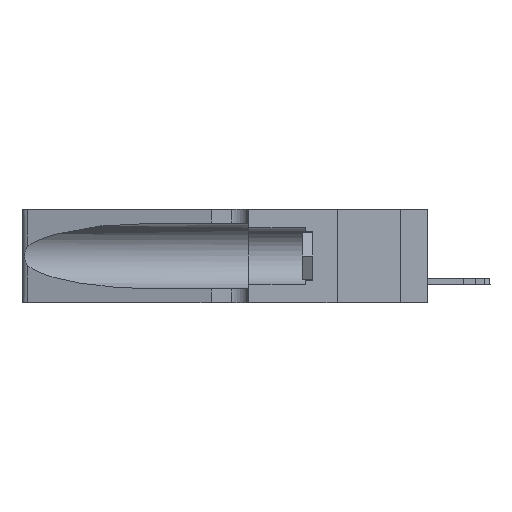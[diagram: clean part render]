
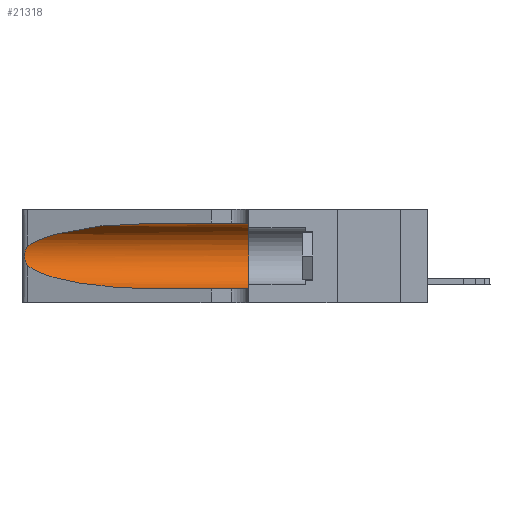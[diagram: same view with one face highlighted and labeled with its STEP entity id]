
A CAD part, left-side view. The second image highlights one B-rep face of the part: STEP entity #21318.
In plain terms, the highlighted cylindrical face has radius 3.308 mm (diameter 6.617 mm), a partial arc.
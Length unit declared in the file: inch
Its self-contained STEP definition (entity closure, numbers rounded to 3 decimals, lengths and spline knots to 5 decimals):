
#778 = DIRECTION ( 'NONE',  ( 0., 0., -1. ) ) ;
#1461 = ORIENTED_EDGE ( 'NONE', *, *, #19994, .F. ) ;
#2462 = CARTESIAN_POINT ( 'NONE',  ( 0.25555, 1.22994, 0.2215 ) ) ;
#2542 = EDGE_LOOP ( 'NONE', ( #11237, #21439, #19529, #3447, #18227, #1461 ) ) ;
#3447 = ORIENTED_EDGE ( 'NONE', *, *, #7201, .T. ) ;
#3636 =( BOUNDED_CURVE ( )  B_SPLINE_CURVE ( 3, ( #21486, #7838, #14524, #28552 ),
 .UNSPECIFIED., .F., .T. ) 
 B_SPLINE_CURVE_WITH_KNOTS ( ( 4, 4 ),
 ( 3.44316, 4.71239 ),
 .UNSPECIFIED. ) 
 CURVE ( )  GEOMETRIC_REPRESENTATION_ITEM ( )  RATIONAL_B_SPLINE_CURVE ( ( 1., 0.87, 0.87, 1. ) ) 
 REPRESENTATION_ITEM ( '' )  );
#3967 = CARTESIAN_POINT ( 'NONE',  ( 0.1305, 1.61858, 0.05475 ) ) ;
#4089 = VECTOR ( 'NONE', #28942, 39.37008 ) ;
#4454 = CARTESIAN_POINT ( 'NONE',  ( 0.26075, 1.23896, 0.19203 ) ) ;
#4654 = CARTESIAN_POINT ( 'NONE',  ( 0.25856, 1.23593, 0.16098 ) ) ;
#5069 = CARTESIAN_POINT ( 'NONE',  ( 0.1305, 1.61858, 0.185 ) ) ;
#5855 = EDGE_CURVE ( 'NONE', #16248, #21308, #26075, .T. ) ;
#6386 = DIRECTION ( 'NONE',  ( 0., 0., 1. ) ) ;
#6632 = CARTESIAN_POINT ( 'NONE',  ( 0.25555, 1.22993, 0.14849 ) ) ;
#6723 = CARTESIAN_POINT ( 'NONE',  ( 0.25487, 1.22718, 0.14631 ) ) ;
#6805 = CARTESIAN_POINT ( 'NONE',  ( 0.25639, 1.23184, 0.21858 ) ) ;
#7201 = EDGE_CURVE ( 'NONE', #9425, #27850, #24384, .T. ) ;
#7838 = CARTESIAN_POINT ( 'NONE',  ( 0.2373, 1.15595, 0.08982 ) ) ;
#8885 = DIRECTION ( 'NONE',  ( 0., -1., 0. ) ) ;
#9065 = CARTESIAN_POINT ( 'NONE',  ( 0.26075, 1.23896, 0.178 ) ) ;
#9425 = VERTEX_POINT ( 'NONE', #17817 ) ;
#10234 = CARTESIAN_POINT ( 'NONE',  ( 0.1305, 0.72297, 0.31525 ) ) ;
#10511 = FACE_OUTER_BOUND ( 'NONE', #2542, .T. ) ;
#11189 = CARTESIAN_POINT ( 'NONE',  ( 0.26017, 1.23833, 0.17102 ) ) ;
#11237 = ORIENTED_EDGE ( 'NONE', *, *, #5855, .T. ) ;
#11334 = LINE ( 'NONE', #22161, #24162 ) ;
#11467 = CARTESIAN_POINT ( 'NONE',  ( 0.25487, 1.22718, 0.22369 ) ) ;
#12929 = B_SPLINE_CURVE_WITH_KNOTS ( 'NONE', 3,
 ( #11467, #2462, #6805, #24854, #22745, #22837, #4454, #9065, #11189, #4654, #27420, #28531, #6632, #6723 ),
 .UNSPECIFIED., .F., .F.,
 ( 4, 2, 2, 2, 2, 2, 4 ),
 ( 0., 0.00027, 0.00053, 0.00107, 0.0016, 0.00187, 0.00214 ),
 .UNSPECIFIED. ) ;
#13054 = DIRECTION ( 'NONE',  ( 0., 1., 0. ) ) ;
#13396 = VERTEX_POINT ( 'NONE', #27294 ) ;
#14204 = CARTESIAN_POINT ( 'NONE',  ( 0.25487, 1.22718, 0.22369 ) ) ;
#14524 = CARTESIAN_POINT ( 'NONE',  ( 0.18966, 0.96281, 0.05475 ) ) ;
#15119 = CARTESIAN_POINT ( 'NONE',  ( 0.25487, 1.22718, 0.22369 ) ) ;
#15885 = CARTESIAN_POINT ( 'NONE',  ( 0.1305, 0.72297, 0.31525 ) ) ;
#16248 = VERTEX_POINT ( 'NONE', #15885 ) ;
#16479 = DIRECTION ( 'NONE',  ( 0., -1., 0. ) ) ;
#16661 = EDGE_CURVE ( 'NONE', #17924, #27850, #25349, .T. ) ;
#17817 = CARTESIAN_POINT ( 'NONE',  ( 0.1305, 0.72297, 0.05475 ) ) ;
#17924 = VERTEX_POINT ( 'NONE', #22054 ) ;
#18227 = ORIENTED_EDGE ( 'NONE', *, *, #16661, .F. ) ;
#18830 = AXIS2_PLACEMENT_3D ( 'NONE', #26690, #13054, #6386 ) ;
#19529 = ORIENTED_EDGE ( 'NONE', *, *, #23996, .T. ) ;
#19994 = EDGE_CURVE ( 'NONE', #16248, #17924, #11334, .T. ) ;
#21308 = VERTEX_POINT ( 'NONE', #14204 ) ;
#21318 = ADVANCED_FACE ( 'NONE', ( #10511 ), #22322, .F. ) ;
#21439 = ORIENTED_EDGE ( 'NONE', *, *, #25933, .T. ) ;
#21486 = CARTESIAN_POINT ( 'NONE',  ( 0.25487, 1.22718, 0.14631 ) ) ;
#21908 = CARTESIAN_POINT ( 'NONE',  ( 0.18966, 0.96281, 0.31525 ) ) ;
#22054 = CARTESIAN_POINT ( 'NONE',  ( 0.1305, 0.35, 0.31525 ) ) ;
#22161 = CARTESIAN_POINT ( 'NONE',  ( 0.1305, 1.61858, 0.31525 ) ) ;
#22322 = CYLINDRICAL_SURFACE ( 'NONE', #27533, 0.13025 ) ;
#22745 = CARTESIAN_POINT ( 'NONE',  ( 0.25854, 1.2359, 0.20912 ) ) ;
#22837 = CARTESIAN_POINT ( 'NONE',  ( 0.26018, 1.23835, 0.19895 ) ) ;
#23612 = CARTESIAN_POINT ( 'NONE',  ( 0.1305, 0.35, 0.05475 ) ) ;
#23996 = EDGE_CURVE ( 'NONE', #13396, #9425, #3636, .T. ) ;
#24162 = VECTOR ( 'NONE', #8885, 39.37008 ) ;
#24384 = LINE ( 'NONE', #3967, #4089 ) ;
#24854 = CARTESIAN_POINT ( 'NONE',  ( 0.25787, 1.23484, 0.2124 ) ) ;
#25349 = CIRCLE ( 'NONE', #18830, 0.13025 ) ;
#25933 = EDGE_CURVE ( 'NONE', #21308, #13396, #12929, .T. ) ;
#26075 =( BOUNDED_CURVE ( )  B_SPLINE_CURVE ( 3, ( #10234, #21908, #28781, #15119 ),
 .UNSPECIFIED., .F., .F. ) 
 B_SPLINE_CURVE_WITH_KNOTS ( ( 4, 4 ),
 ( 1.5708, 2.84003 ),
 .UNSPECIFIED. ) 
 CURVE ( )  GEOMETRIC_REPRESENTATION_ITEM ( )  RATIONAL_B_SPLINE_CURVE ( ( 1., 0.87, 0.87, 1. ) ) 
 REPRESENTATION_ITEM ( '' )  );
#26690 = CARTESIAN_POINT ( 'NONE',  ( 0.1305, 0.35, 0.185 ) ) ;
#27294 = CARTESIAN_POINT ( 'NONE',  ( 0.25487, 1.22718, 0.14631 ) ) ;
#27420 = CARTESIAN_POINT ( 'NONE',  ( 0.25789, 1.23486, 0.15765 ) ) ;
#27533 = AXIS2_PLACEMENT_3D ( 'NONE', #5069, #16479, #778 ) ;
#27850 = VERTEX_POINT ( 'NONE', #23612 ) ;
#28531 = CARTESIAN_POINT ( 'NONE',  ( 0.25639, 1.23186, 0.15144 ) ) ;
#28552 = CARTESIAN_POINT ( 'NONE',  ( 0.1305, 0.72297, 0.05475 ) ) ;
#28781 = CARTESIAN_POINT ( 'NONE',  ( 0.2373, 1.15595, 0.28018 ) ) ;
#28942 = DIRECTION ( 'NONE',  ( 0., -1., 0. ) ) ;
